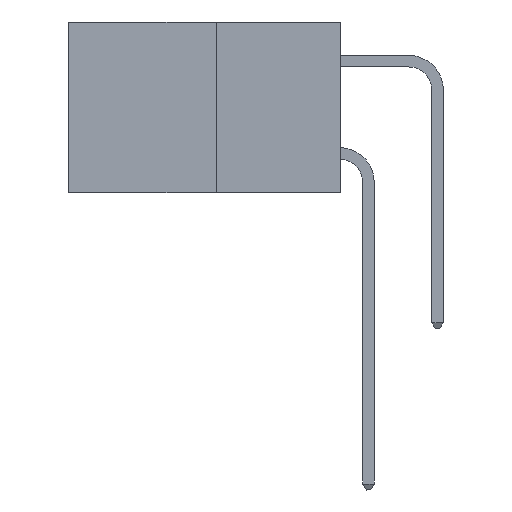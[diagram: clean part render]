
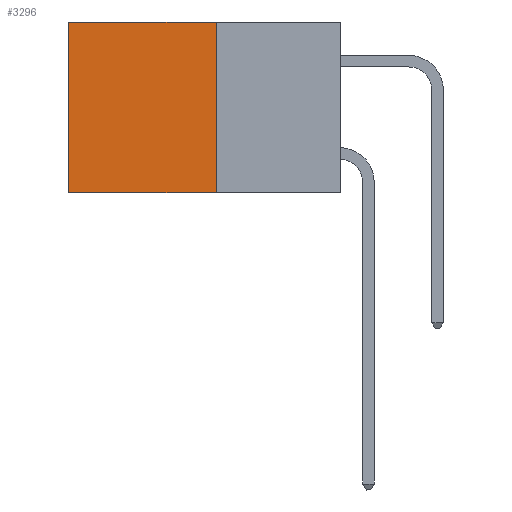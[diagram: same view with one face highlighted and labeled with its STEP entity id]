
A CAD part, left-side view. The second image highlights one B-rep face of the part: STEP entity #3296.
In plain terms, the highlighted planar face has unit normal (-1, 0, 0).
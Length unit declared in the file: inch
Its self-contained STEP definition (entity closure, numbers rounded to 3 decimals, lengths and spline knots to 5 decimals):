
#374 = ORIENTED_EDGE ( 'NONE', *, *, #28286, .T. ) ;
#828 = VERTEX_POINT ( 'NONE', #27825 ) ;
#1307 = CARTESIAN_POINT ( 'NONE',  ( 0.277, 0.59, -0.37 ) ) ;
#1339 = EDGE_CURVE ( 'NONE', #12009, #1455, #6389, .T. ) ;
#1361 = CARTESIAN_POINT ( 'NONE',  ( 0.277, 0.27, -0.37 ) ) ;
#1455 = VERTEX_POINT ( 'NONE', #22866 ) ;
#1523 = CARTESIAN_POINT ( 'NONE',  ( 0.277, 0.27, -0.37 ) ) ;
#2726 = FACE_OUTER_BOUND ( 'NONE', #3467, .T. ) ;
#3296 = ADVANCED_FACE ( 'NONE', ( #2726 ), #19072, .F. ) ;
#3467 = EDGE_LOOP ( 'NONE', ( #374, #12021, #3977, #26822 ) ) ;
#3977 = ORIENTED_EDGE ( 'NONE', *, *, #20432, .F. ) ;
#4740 = VECTOR ( 'NONE', #21565, 39.37008 ) ;
#6185 = CARTESIAN_POINT ( 'NONE',  ( 0.277, 0.27, -0.37 ) ) ;
#6389 = LINE ( 'NONE', #6185, #18134 ) ;
#8612 = EDGE_CURVE ( 'NONE', #23569, #828, #10030, .T. ) ;
#10030 = LINE ( 'NONE', #21109, #15236 ) ;
#12009 = VERTEX_POINT ( 'NONE', #1361 ) ;
#12021 = ORIENTED_EDGE ( 'NONE', *, *, #1339, .F. ) ;
#15236 = VECTOR ( 'NONE', #18333, 39.37008 ) ;
#15825 = DIRECTION ( 'NONE',  ( 0., 1., 0. ) ) ;
#16171 = DIRECTION ( 'NONE',  ( 0., 0., -1. ) ) ;
#16197 = DIRECTION ( 'NONE',  ( 1., 0., 0. ) ) ;
#16996 = CARTESIAN_POINT ( 'NONE',  ( 0.277, 0.27, -0.37 ) ) ;
#18134 = VECTOR ( 'NONE', #15825, 39.37008 ) ;
#18333 = DIRECTION ( 'NONE',  ( 0., 1., 0. ) ) ;
#19072 = PLANE ( 'NONE',  #28371 ) ;
#19109 = DIRECTION ( 'NONE',  ( 0., 0., -1. ) ) ;
#20432 = EDGE_CURVE ( 'NONE', #23569, #12009, #22423, .T. ) ;
#21109 = CARTESIAN_POINT ( 'NONE',  ( 0.277, 0.27, 0. ) ) ;
#21565 = DIRECTION ( 'NONE',  ( 0., 0., -1. ) ) ;
#22423 = LINE ( 'NONE', #1523, #4740 ) ;
#22866 = CARTESIAN_POINT ( 'NONE',  ( 0.277, 0.59, -0.37 ) ) ;
#23300 = LINE ( 'NONE', #1307, #28478 ) ;
#23318 = CARTESIAN_POINT ( 'NONE',  ( 0.277, 0.27, 0. ) ) ;
#23569 = VERTEX_POINT ( 'NONE', #23318 ) ;
#26822 = ORIENTED_EDGE ( 'NONE', *, *, #8612, .T. ) ;
#27825 = CARTESIAN_POINT ( 'NONE',  ( 0.277, 0.59, 0. ) ) ;
#28286 = EDGE_CURVE ( 'NONE', #828, #1455, #23300, .T. ) ;
#28371 = AXIS2_PLACEMENT_3D ( 'NONE', #16996, #16197, #16171 ) ;
#28478 = VECTOR ( 'NONE', #19109, 39.37008 ) ;
